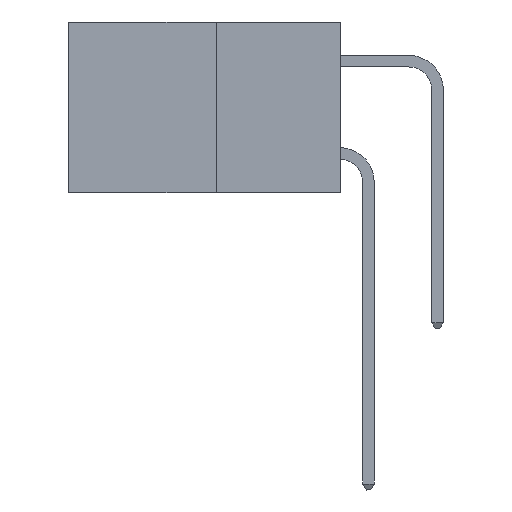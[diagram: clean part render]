
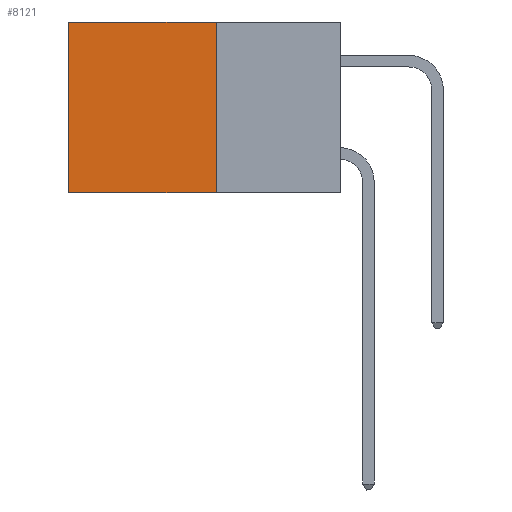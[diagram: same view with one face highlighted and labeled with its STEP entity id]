
A CAD part, left-side view. The second image highlights one B-rep face of the part: STEP entity #8121.
In plain terms, the highlighted planar face has unit normal (-1, 0, 0).
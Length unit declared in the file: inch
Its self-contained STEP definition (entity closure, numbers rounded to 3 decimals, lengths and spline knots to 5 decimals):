
#65 = VERTEX_POINT ( 'NONE', #5505 ) ;
#1044 = EDGE_CURVE ( 'NONE', #13859, #2337, #3650, .T. ) ;
#1169 = FACE_OUTER_BOUND ( 'NONE', #2138, .T. ) ;
#1559 = DIRECTION ( 'NONE',  ( 0., 1., 0. ) ) ;
#1842 = ORIENTED_EDGE ( 'NONE', *, *, #4938, .T. ) ;
#2013 = ORIENTED_EDGE ( 'NONE', *, *, #1044, .F. ) ;
#2138 = EDGE_LOOP ( 'NONE', ( #11613, #16126, #2013, #1842 ) ) ;
#2337 = VERTEX_POINT ( 'NONE', #10023 ) ;
#2408 = EDGE_CURVE ( 'NONE', #18371, #65, #17242, .T. ) ;
#2602 = CARTESIAN_POINT ( 'NONE',  ( 0.277, 0.27, -0.37 ) ) ;
#3346 = CARTESIAN_POINT ( 'NONE',  ( 0.277, 0.27, -0.37 ) ) ;
#3491 = VECTOR ( 'NONE', #1559, 39.37008 ) ;
#3650 = LINE ( 'NONE', #2602, #22018 ) ;
#4938 = EDGE_CURVE ( 'NONE', #13859, #18371, #13009, .T. ) ;
#5121 = DIRECTION ( 'NONE',  ( 0., 0., -1. ) ) ;
#5469 = CARTESIAN_POINT ( 'NONE',  ( 0.277, 0.27, 0. ) ) ;
#5505 = CARTESIAN_POINT ( 'NONE',  ( 0.277, 0.59, -0.37 ) ) ;
#7801 = VECTOR ( 'NONE', #13446, 39.37008 ) ;
#8121 = ADVANCED_FACE ( 'NONE', ( #1169 ), #12272, .F. ) ;
#10023 = CARTESIAN_POINT ( 'NONE',  ( 0.277, 0.27, -0.37 ) ) ;
#10453 = CARTESIAN_POINT ( 'NONE',  ( 0.277, 0.27, -0.37 ) ) ;
#11613 = ORIENTED_EDGE ( 'NONE', *, *, #2408, .T. ) ;
#11983 = CARTESIAN_POINT ( 'NONE',  ( 0.277, 0.59, -0.37 ) ) ;
#12272 = PLANE ( 'NONE',  #22613 ) ;
#12305 = EDGE_CURVE ( 'NONE', #2337, #65, #18808, .T. ) ;
#13001 = VECTOR ( 'NONE', #15825, 39.37008 ) ;
#13009 = LINE ( 'NONE', #22878, #3491 ) ;
#13446 = DIRECTION ( 'NONE',  ( 0., 0., -1. ) ) ;
#13859 = VERTEX_POINT ( 'NONE', #5469 ) ;
#14317 = CARTESIAN_POINT ( 'NONE',  ( 0.277, 0.59, 0. ) ) ;
#15810 = DIRECTION ( 'NONE',  ( 1., 0., 0. ) ) ;
#15825 = DIRECTION ( 'NONE',  ( 0., 1., 0. ) ) ;
#16126 = ORIENTED_EDGE ( 'NONE', *, *, #12305, .F. ) ;
#17242 = LINE ( 'NONE', #11983, #7801 ) ;
#17610 = DIRECTION ( 'NONE',  ( 0., 0., -1. ) ) ;
#18371 = VERTEX_POINT ( 'NONE', #14317 ) ;
#18808 = LINE ( 'NONE', #10453, #13001 ) ;
#22018 = VECTOR ( 'NONE', #17610, 39.37008 ) ;
#22613 = AXIS2_PLACEMENT_3D ( 'NONE', #3346, #15810, #5121 ) ;
#22878 = CARTESIAN_POINT ( 'NONE',  ( 0.277, 0.27, 0. ) ) ;
